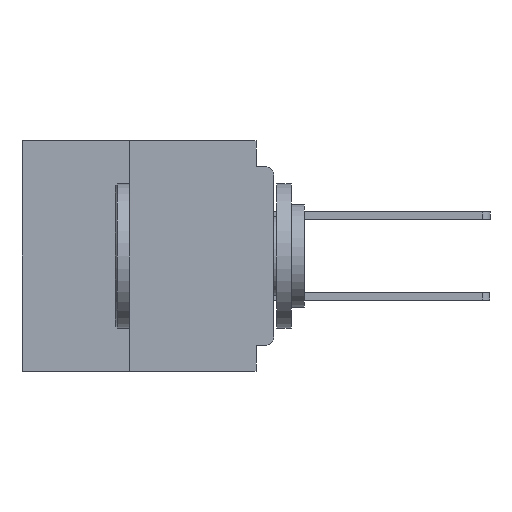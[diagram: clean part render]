
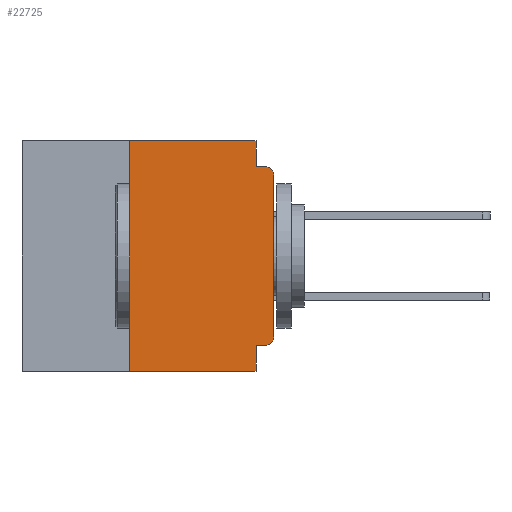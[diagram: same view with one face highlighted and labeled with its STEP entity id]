
A CAD part, left-side view. The second image highlights one B-rep face of the part: STEP entity #22725.
In plain terms, the highlighted planar face has unit normal (-1, 0, 0).
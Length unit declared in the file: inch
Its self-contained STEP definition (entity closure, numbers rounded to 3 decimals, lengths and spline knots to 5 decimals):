
#1619 = EDGE_CURVE ( 'NONE', #21892, #40490, #33803, .T. ) ;
#3480 = VERTEX_POINT ( 'NONE', #52615 ) ;
#4034 = VECTOR ( 'NONE', #52845, 39.37008 ) ;
#5880 = VECTOR ( 'NONE', #56122, 39.37008 ) ;
#5901 = CARTESIAN_POINT ( 'NONE',  ( 0., 0.015, -0.06 ) ) ;
#6434 = DIRECTION ( 'NONE',  ( 1., 0., 0. ) ) ;
#8741 = CARTESIAN_POINT ( 'NONE',  ( 0., 0.031, -0.4 ) ) ;
#9084 = CARTESIAN_POINT ( 'NONE',  ( 0., 0., 0. ) ) ;
#10014 = LINE ( 'NONE', #51795, #5880 ) ;
#10314 = DIRECTION ( 'NONE',  ( 0., 0., -1. ) ) ;
#10648 = VECTOR ( 'NONE', #50628, 39.37008 ) ;
#10665 = PLANE ( 'NONE',  #53004 ) ;
#11489 = EDGE_CURVE ( 'NONE', #37509, #36109, #27802, .T. ) ;
#11519 = ORIENTED_EDGE ( 'NONE', *, *, #28385, .T. ) ;
#12917 = EDGE_CURVE ( 'NONE', #3480, #40704, #47285, .T. ) ;
#14827 = CARTESIAN_POINT ( 'NONE',  ( 0., 0.015, -0.34 ) ) ;
#15644 = CARTESIAN_POINT ( 'NONE',  ( 0., 0.031, -0.045 ) ) ;
#16467 = ORIENTED_EDGE ( 'NONE', *, *, #47228, .F. ) ;
#16672 = VERTEX_POINT ( 'NONE', #34581 ) ;
#18564 = EDGE_CURVE ( 'NONE', #51981, #33728, #53007, .T. ) ;
#18580 = ORIENTED_EDGE ( 'NONE', *, *, #31819, .T. ) ;
#19206 = DIRECTION ( 'NONE',  ( 0., 0., -1. ) ) ;
#20100 = CARTESIAN_POINT ( 'NONE',  ( 0., 0.031, -0.355 ) ) ;
#21497 = CARTESIAN_POINT ( 'NONE',  ( 0., 0.031, 0. ) ) ;
#21892 = VERTEX_POINT ( 'NONE', #25157 ) ;
#22725 = ADVANCED_FACE ( 'NONE', ( #43904 ), #10665, .F. ) ;
#23717 = EDGE_CURVE ( 'NONE', #40704, #16672, #10014, .T. ) ;
#24623 = CARTESIAN_POINT ( 'NONE',  ( 0., 0.031, -0.4 ) ) ;
#25157 = CARTESIAN_POINT ( 'NONE',  ( 0., 0.015, -0.355 ) ) ;
#25252 = EDGE_CURVE ( 'NONE', #40490, #52431, #43756, .T. ) ;
#25820 = CARTESIAN_POINT ( 'NONE',  ( 0., 0., -0.34 ) ) ;
#27245 = LINE ( 'NONE', #53022, #4034 ) ;
#27802 = LINE ( 'NONE', #31199, #49343 ) ;
#27968 = ORIENTED_EDGE ( 'NONE', *, *, #23717, .F. ) ;
#28385 = EDGE_CURVE ( 'NONE', #3480, #52431, #27245, .T. ) ;
#29587 = VECTOR ( 'NONE', #56196, 39.37008 ) ;
#29804 = CIRCLE ( 'NONE', #43958, 0.015 ) ;
#31199 = CARTESIAN_POINT ( 'NONE',  ( 0., 0., -0.045 ) ) ;
#31819 = EDGE_CURVE ( 'NONE', #21892, #51981, #44460, .T. ) ;
#32557 = CARTESIAN_POINT ( 'NONE',  ( 0., 0.437, 0. ) ) ;
#32912 = ORIENTED_EDGE ( 'NONE', *, *, #18564, .T. ) ;
#33728 = VERTEX_POINT ( 'NONE', #34133 ) ;
#33803 = LINE ( 'NONE', #49997, #10648 ) ;
#34133 = CARTESIAN_POINT ( 'NONE',  ( 0., 0., -0.06 ) ) ;
#34266 = AXIS2_PLACEMENT_3D ( 'NONE', #14827, #45099, #19206 ) ;
#34450 = CARTESIAN_POINT ( 'NONE',  ( 0., 0.015, -0.045 ) ) ;
#34524 = VECTOR ( 'NONE', #41005, 39.37008 ) ;
#34581 = CARTESIAN_POINT ( 'NONE',  ( 0., 0.031, 0. ) ) ;
#35139 = DIRECTION ( 'NONE',  ( 0., 0., 1. ) ) ;
#36109 = VERTEX_POINT ( 'NONE', #34450 ) ;
#36327 = DIRECTION ( 'NONE',  ( -1., 0., 0. ) ) ;
#36871 = DIRECTION ( 'NONE',  ( 0., 0., -1. ) ) ;
#37350 = EDGE_CURVE ( 'NONE', #33728, #36109, #29804, .T. ) ;
#37509 = VERTEX_POINT ( 'NONE', #15644 ) ;
#38544 = DIRECTION ( 'NONE',  ( 0., 0., -1. ) ) ;
#40490 = VERTEX_POINT ( 'NONE', #20100 ) ;
#40704 = VERTEX_POINT ( 'NONE', #47473 ) ;
#41005 = DIRECTION ( 'NONE',  ( 0., 0., 1. ) ) ;
#41582 = VECTOR ( 'NONE', #35139, 39.37008 ) ;
#42193 = ORIENTED_EDGE ( 'NONE', *, *, #1619, .F. ) ;
#43756 = LINE ( 'NONE', #8741, #29587 ) ;
#43904 = FACE_OUTER_BOUND ( 'NONE', #54638, .T. ) ;
#43958 = AXIS2_PLACEMENT_3D ( 'NONE', #5901, #36327, #10314 ) ;
#44010 = DIRECTION ( 'NONE',  ( 0., -1., 0. ) ) ;
#44403 = ORIENTED_EDGE ( 'NONE', *, *, #37350, .T. ) ;
#44460 = CIRCLE ( 'NONE', #34266, 0.015 ) ;
#45099 = DIRECTION ( 'NONE',  ( -1., 0., 0. ) ) ;
#45358 = CARTESIAN_POINT ( 'NONE',  ( 0., 0.25, -0.4 ) ) ;
#47037 = ORIENTED_EDGE ( 'NONE', *, *, #11489, .F. ) ;
#47228 = EDGE_CURVE ( 'NONE', #16672, #37509, #50167, .T. ) ;
#47285 = LINE ( 'NONE', #45358, #34524 ) ;
#47473 = CARTESIAN_POINT ( 'NONE',  ( 0., 0.25, 0. ) ) ;
#47809 = ORIENTED_EDGE ( 'NONE', *, *, #25252, .F. ) ;
#48824 = VECTOR ( 'NONE', #38544, 39.37008 ) ;
#49343 = VECTOR ( 'NONE', #44010, 39.37008 ) ;
#49997 = CARTESIAN_POINT ( 'NONE',  ( 0., 0., -0.355 ) ) ;
#50167 = LINE ( 'NONE', #21497, #48824 ) ;
#50628 = DIRECTION ( 'NONE',  ( 0., 1., 0. ) ) ;
#51795 = CARTESIAN_POINT ( 'NONE',  ( 0., 0.437, 0. ) ) ;
#51981 = VERTEX_POINT ( 'NONE', #25820 ) ;
#52431 = VERTEX_POINT ( 'NONE', #24623 ) ;
#52615 = CARTESIAN_POINT ( 'NONE',  ( 0., 0.25, -0.4 ) ) ;
#52845 = DIRECTION ( 'NONE',  ( 0., -1., 0. ) ) ;
#53004 = AXIS2_PLACEMENT_3D ( 'NONE', #32557, #6434, #36871 ) ;
#53007 = LINE ( 'NONE', #9084, #41582 ) ;
#53022 = CARTESIAN_POINT ( 'NONE',  ( 0., 0.437, -0.4 ) ) ;
#54638 = EDGE_LOOP ( 'NONE', ( #32912, #44403, #47037, #16467, #27968, #55328, #11519, #47809, #42193, #18580 ) ) ;
#55328 = ORIENTED_EDGE ( 'NONE', *, *, #12917, .F. ) ;
#56122 = DIRECTION ( 'NONE',  ( 0., -1., 0. ) ) ;
#56196 = DIRECTION ( 'NONE',  ( 0., 0., -1. ) ) ;
